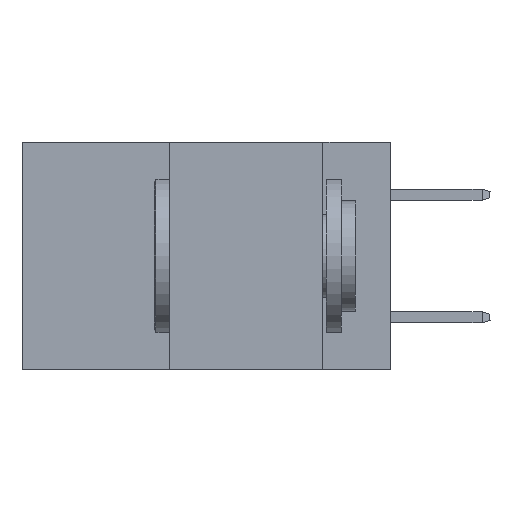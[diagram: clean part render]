
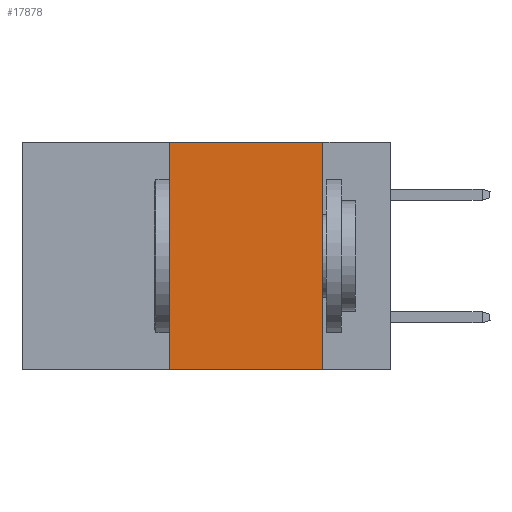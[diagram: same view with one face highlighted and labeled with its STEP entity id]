
A CAD part, left-side view. The second image highlights one B-rep face of the part: STEP entity #17878.
In plain terms, the highlighted planar face has unit normal (-1, 0, 0).
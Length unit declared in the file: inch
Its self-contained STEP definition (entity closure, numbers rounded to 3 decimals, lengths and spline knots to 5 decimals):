
#626 = LINE ( 'NONE', #2587, #7367 ) ;
#819 = EDGE_CURVE ( 'NONE', #15406, #15232, #17842, .T. ) ;
#1477 = PLANE ( 'NONE',  #7240 ) ;
#2587 = CARTESIAN_POINT ( 'NONE',  ( 0., 0.6, 0. ) ) ;
#3859 = CARTESIAN_POINT ( 'NONE',  ( 0., 0.36, 0. ) ) ;
#4230 = EDGE_CURVE ( 'NONE', #16981, #15232, #4970, .T. ) ;
#4278 = FACE_OUTER_BOUND ( 'NONE', #11558, .T. ) ;
#4543 = VECTOR ( 'NONE', #12237, 39.37008 ) ;
#4586 = DIRECTION ( 'NONE',  ( 0., 0., -1. ) ) ;
#4970 = LINE ( 'NONE', #13625, #15974 ) ;
#7240 = AXIS2_PLACEMENT_3D ( 'NONE', #11861, #13271, #4586 ) ;
#7367 = VECTOR ( 'NONE', #12821, 39.37008 ) ;
#8579 = EDGE_CURVE ( 'NONE', #15406, #18192, #8943, .T. ) ;
#8887 = EDGE_CURVE ( 'NONE', #18192, #16981, #626, .T. ) ;
#8943 = LINE ( 'NONE', #10815, #4543 ) ;
#9924 = CARTESIAN_POINT ( 'NONE',  ( 0., 0.6, -0.37 ) ) ;
#10200 = ORIENTED_EDGE ( 'NONE', *, *, #819, .T. ) ;
#10815 = CARTESIAN_POINT ( 'NONE',  ( 0., 0.36, 0. ) ) ;
#11558 = EDGE_LOOP ( 'NONE', ( #15218, #16731, #13355, #10200 ) ) ;
#11815 = DIRECTION ( 'NONE',  ( 0., -1., 0. ) ) ;
#11861 = CARTESIAN_POINT ( 'NONE',  ( 0., 0.6, 0. ) ) ;
#11941 = CARTESIAN_POINT ( 'NONE',  ( 0., 0.36, -0.37 ) ) ;
#12201 = CARTESIAN_POINT ( 'NONE',  ( 0., 0.11, -0.37 ) ) ;
#12237 = DIRECTION ( 'NONE',  ( 0., 0., 1. ) ) ;
#12821 = DIRECTION ( 'NONE',  ( 0., -1., 0. ) ) ;
#13271 = DIRECTION ( 'NONE',  ( 1., 0., 0. ) ) ;
#13355 = ORIENTED_EDGE ( 'NONE', *, *, #8579, .F. ) ;
#13606 = DIRECTION ( 'NONE',  ( 0., 0., -1. ) ) ;
#13625 = CARTESIAN_POINT ( 'NONE',  ( 0., 0.11, 0. ) ) ;
#13973 = CARTESIAN_POINT ( 'NONE',  ( 0., 0.11, 0. ) ) ;
#14564 = VECTOR ( 'NONE', #11815, 39.37008 ) ;
#15218 = ORIENTED_EDGE ( 'NONE', *, *, #4230, .F. ) ;
#15232 = VERTEX_POINT ( 'NONE', #12201 ) ;
#15406 = VERTEX_POINT ( 'NONE', #11941 ) ;
#15974 = VECTOR ( 'NONE', #13606, 39.37008 ) ;
#16731 = ORIENTED_EDGE ( 'NONE', *, *, #8887, .F. ) ;
#16981 = VERTEX_POINT ( 'NONE', #13973 ) ;
#17842 = LINE ( 'NONE', #9924, #14564 ) ;
#17878 = ADVANCED_FACE ( 'NONE', ( #4278 ), #1477, .F. ) ;
#18192 = VERTEX_POINT ( 'NONE', #3859 ) ;
